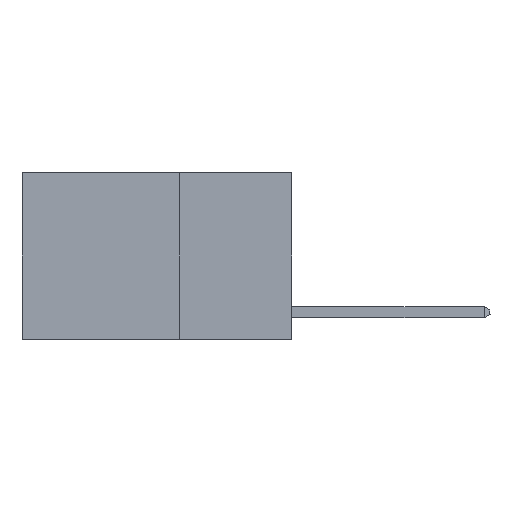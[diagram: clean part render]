
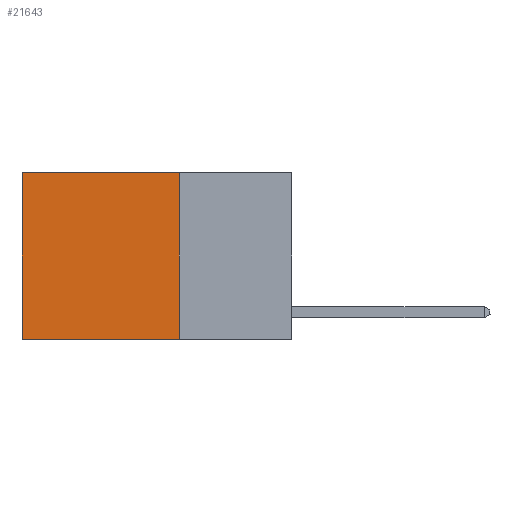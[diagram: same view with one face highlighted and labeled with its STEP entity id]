
A CAD part, left-side view. The second image highlights one B-rep face of the part: STEP entity #21643.
In plain terms, the highlighted planar face has unit normal (-1, 0, 0).
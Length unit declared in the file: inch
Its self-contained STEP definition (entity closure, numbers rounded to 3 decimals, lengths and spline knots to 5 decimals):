
#517 = EDGE_CURVE ( 'NONE', #17976, #26051, #4584, .T. ) ;
#1568 = VECTOR ( 'NONE', #8422, 39.37008 ) ;
#2335 = CARTESIAN_POINT ( 'NONE',  ( 0.2625, 0.6, -0.37 ) ) ;
#3666 = LINE ( 'NONE', #9722, #8723 ) ;
#4430 = CARTESIAN_POINT ( 'NONE',  ( 0.2625, 0.25, 0. ) ) ;
#4584 = LINE ( 'NONE', #9452, #10266 ) ;
#5236 = PLANE ( 'NONE',  #18501 ) ;
#5254 = EDGE_CURVE ( 'NONE', #17976, #18141, #16840, .T. ) ;
#5328 = DIRECTION ( 'NONE',  ( 1., 0., 0. ) ) ;
#5405 = FACE_OUTER_BOUND ( 'NONE', #10193, .T. ) ;
#6176 = CARTESIAN_POINT ( 'NONE',  ( 0.2625, 0.6, 0. ) ) ;
#7063 = CARTESIAN_POINT ( 'NONE',  ( 0.2625, 0.25, -0.37 ) ) ;
#7332 = LINE ( 'NONE', #6176, #1568 ) ;
#7362 = EDGE_CURVE ( 'NONE', #26051, #13484, #7332, .T. ) ;
#8422 = DIRECTION ( 'NONE',  ( 0., 0., -1. ) ) ;
#8723 = VECTOR ( 'NONE', #11884, 39.37008 ) ;
#9452 = CARTESIAN_POINT ( 'NONE',  ( 0.2625, 0.25, 0. ) ) ;
#9722 = CARTESIAN_POINT ( 'NONE',  ( 0.2625, 0.25, -0.37 ) ) ;
#9998 = CARTESIAN_POINT ( 'NONE',  ( 0.2625, 0.25, 0. ) ) ;
#10193 = EDGE_LOOP ( 'NONE', ( #17573, #27048, #22297, #13326 ) ) ;
#10266 = VECTOR ( 'NONE', #22275, 39.37008 ) ;
#11884 = DIRECTION ( 'NONE',  ( 0., 1., 0. ) ) ;
#11889 = EDGE_CURVE ( 'NONE', #18141, #13484, #3666, .T. ) ;
#12162 = DIRECTION ( 'NONE',  ( 0., 0., -1. ) ) ;
#13326 = ORIENTED_EDGE ( 'NONE', *, *, #517, .T. ) ;
#13484 = VERTEX_POINT ( 'NONE', #2335 ) ;
#16840 = LINE ( 'NONE', #9998, #27497 ) ;
#17573 = ORIENTED_EDGE ( 'NONE', *, *, #7362, .T. ) ;
#17976 = VERTEX_POINT ( 'NONE', #4430 ) ;
#18141 = VERTEX_POINT ( 'NONE', #7063 ) ;
#18153 = CARTESIAN_POINT ( 'NONE',  ( 0.2625, 0.25, 0. ) ) ;
#18501 = AXIS2_PLACEMENT_3D ( 'NONE', #18153, #5328, #20288 ) ;
#19181 = CARTESIAN_POINT ( 'NONE',  ( 0.2625, 0.6, 0. ) ) ;
#20288 = DIRECTION ( 'NONE',  ( 0., 0., -1. ) ) ;
#21643 = ADVANCED_FACE ( 'NONE', ( #5405 ), #5236, .F. ) ;
#22275 = DIRECTION ( 'NONE',  ( 0., 1., 0. ) ) ;
#22297 = ORIENTED_EDGE ( 'NONE', *, *, #5254, .F. ) ;
#26051 = VERTEX_POINT ( 'NONE', #19181 ) ;
#27048 = ORIENTED_EDGE ( 'NONE', *, *, #11889, .F. ) ;
#27497 = VECTOR ( 'NONE', #12162, 39.37008 ) ;
